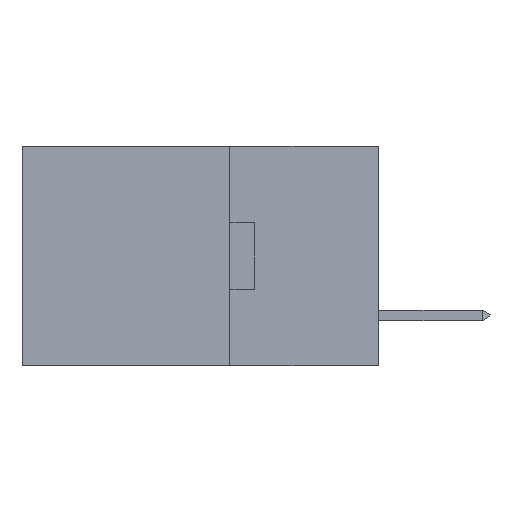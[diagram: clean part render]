
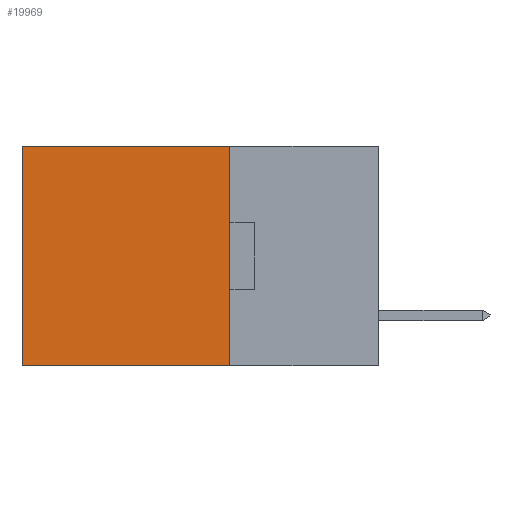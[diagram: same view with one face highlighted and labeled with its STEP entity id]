
A CAD part, left-side view. The second image highlights one B-rep face of the part: STEP entity #19969.
In plain terms, the highlighted planar face has unit normal (-1, 0, 0).
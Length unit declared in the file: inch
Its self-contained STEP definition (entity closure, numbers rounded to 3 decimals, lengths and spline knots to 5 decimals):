
#54 = DIRECTION ( 'NONE',  ( 0., 0., -1. ) ) ;
#752 = EDGE_CURVE ( 'NONE', #2544, #4831, #2526, .T. ) ;
#1304 = ORIENTED_EDGE ( 'NONE', *, *, #22475, .F. ) ;
#2526 = LINE ( 'NONE', #16381, #21694 ) ;
#2544 = VERTEX_POINT ( 'NONE', #20946 ) ;
#3311 = AXIS2_PLACEMENT_3D ( 'NONE', #14537, #18451, #54 ) ;
#4339 = VERTEX_POINT ( 'NONE', #17568 ) ;
#4675 = ORIENTED_EDGE ( 'NONE', *, *, #16619, .F. ) ;
#4724 = EDGE_CURVE ( 'NONE', #4831, #5483, #25423, .T. ) ;
#4831 = VERTEX_POINT ( 'NONE', #24221 ) ;
#5483 = VERTEX_POINT ( 'NONE', #24573 ) ;
#5533 = DIRECTION ( 'NONE',  ( 0., 1., 0. ) ) ;
#8868 = LINE ( 'NONE', #17052, #11331 ) ;
#9542 = CARTESIAN_POINT ( 'NONE',  ( 0.2615, 0.25, -0.37 ) ) ;
#11331 = VECTOR ( 'NONE', #15028, 39.37008 ) ;
#11810 = LINE ( 'NONE', #9542, #17971 ) ;
#12483 = DIRECTION ( 'NONE',  ( 0., 1., 0. ) ) ;
#13344 = ORIENTED_EDGE ( 'NONE', *, *, #752, .T. ) ;
#14537 = CARTESIAN_POINT ( 'NONE',  ( 0.2615, 0.25, -0.37 ) ) ;
#15028 = DIRECTION ( 'NONE',  ( 0., 0., -1. ) ) ;
#16381 = CARTESIAN_POINT ( 'NONE',  ( 0.2615, 0.25, 0. ) ) ;
#16619 = EDGE_CURVE ( 'NONE', #2544, #4339, #8868, .T. ) ;
#16689 = FACE_OUTER_BOUND ( 'NONE', #18205, .T. ) ;
#17052 = CARTESIAN_POINT ( 'NONE',  ( 0.2615, 0.25, -0.37 ) ) ;
#17568 = CARTESIAN_POINT ( 'NONE',  ( 0.2615, 0.25, -0.37 ) ) ;
#17971 = VECTOR ( 'NONE', #5533, 39.37008 ) ;
#17994 = VECTOR ( 'NONE', #25297, 39.37008 ) ;
#18205 = EDGE_LOOP ( 'NONE', ( #25014, #1304, #4675, #13344 ) ) ;
#18451 = DIRECTION ( 'NONE',  ( 1., 0., 0. ) ) ;
#18709 = PLANE ( 'NONE',  #3311 ) ;
#19969 = ADVANCED_FACE ( 'NONE', ( #16689 ), #18709, .F. ) ;
#20946 = CARTESIAN_POINT ( 'NONE',  ( 0.2615, 0.25, 0. ) ) ;
#21694 = VECTOR ( 'NONE', #12483, 39.37008 ) ;
#22475 = EDGE_CURVE ( 'NONE', #4339, #5483, #11810, .T. ) ;
#23684 = CARTESIAN_POINT ( 'NONE',  ( 0.2615, 0.6, -0.37 ) ) ;
#24221 = CARTESIAN_POINT ( 'NONE',  ( 0.2615, 0.6, 0. ) ) ;
#24573 = CARTESIAN_POINT ( 'NONE',  ( 0.2615, 0.6, -0.37 ) ) ;
#25014 = ORIENTED_EDGE ( 'NONE', *, *, #4724, .T. ) ;
#25297 = DIRECTION ( 'NONE',  ( 0., 0., -1. ) ) ;
#25423 = LINE ( 'NONE', #23684, #17994 ) ;
